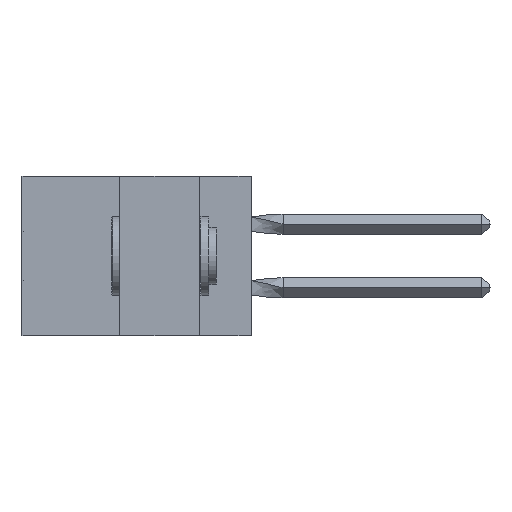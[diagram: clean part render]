
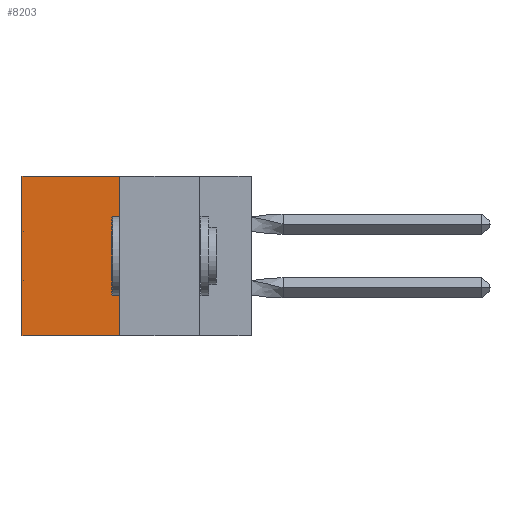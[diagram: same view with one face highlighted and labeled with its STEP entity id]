
A CAD part, left-side view. The second image highlights one B-rep face of the part: STEP entity #8203.
In plain terms, the highlighted planar face has unit normal (-1, 0, 0).
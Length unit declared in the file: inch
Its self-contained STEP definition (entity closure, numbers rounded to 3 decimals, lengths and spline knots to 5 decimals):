
#455 = VECTOR ( 'NONE', #11552, 39.37008 ) ;
#884 = CARTESIAN_POINT ( 'NONE',  ( 0.305, 0.72, -0.5 ) ) ;
#1140 = LINE ( 'NONE', #884, #28678 ) ;
#1660 = VERTEX_POINT ( 'NONE', #36398 ) ;
#2373 = EDGE_CURVE ( 'NONE', #28975, #3886, #28406, .T. ) ;
#2977 = DIRECTION ( 'NONE',  ( 1., 0., 0. ) ) ;
#3886 = VERTEX_POINT ( 'NONE', #41334 ) ;
#4423 = PLANE ( 'NONE',  #13043 ) ;
#5890 = DIRECTION ( 'NONE',  ( 0., 0., -1. ) ) ;
#8203 = ADVANCED_FACE ( 'NONE', ( #32040 ), #4423, .F. ) ;
#9246 = DIRECTION ( 'NONE',  ( 0., 1., 0. ) ) ;
#10403 = CARTESIAN_POINT ( 'NONE',  ( 0.305, 0.413, -0.5 ) ) ;
#11552 = DIRECTION ( 'NONE',  ( 0., 1., 0. ) ) ;
#13043 = AXIS2_PLACEMENT_3D ( 'NONE', #19679, #2977, #5890 ) ;
#13833 = VECTOR ( 'NONE', #9246, 39.37008 ) ;
#17580 = EDGE_CURVE ( 'NONE', #3886, #1660, #1140, .T. ) ;
#18030 = EDGE_LOOP ( 'NONE', ( #36988, #32866, #40586, #39161 ) ) ;
#18140 = LINE ( 'NONE', #10403, #455 ) ;
#18523 = VERTEX_POINT ( 'NONE', #29036 ) ;
#19679 = CARTESIAN_POINT ( 'NONE',  ( 0.305, 0.413, -0.5 ) ) ;
#22125 = CARTESIAN_POINT ( 'NONE',  ( 0.305, 0.413, -0.5 ) ) ;
#23223 = LINE ( 'NONE', #22125, #24782 ) ;
#24782 = VECTOR ( 'NONE', #32631, 39.37008 ) ;
#27350 = EDGE_CURVE ( 'NONE', #18523, #1660, #18140, .T. ) ;
#28406 = LINE ( 'NONE', #42436, #13833 ) ;
#28678 = VECTOR ( 'NONE', #30385, 39.37008 ) ;
#28975 = VERTEX_POINT ( 'NONE', #42535 ) ;
#29036 = CARTESIAN_POINT ( 'NONE',  ( 0.305, 0.413, -0.5 ) ) ;
#30385 = DIRECTION ( 'NONE',  ( 0., 0., -1. ) ) ;
#32040 = FACE_OUTER_BOUND ( 'NONE', #18030, .T. ) ;
#32631 = DIRECTION ( 'NONE',  ( 0., 0., -1. ) ) ;
#32866 = ORIENTED_EDGE ( 'NONE', *, *, #27350, .F. ) ;
#36398 = CARTESIAN_POINT ( 'NONE',  ( 0.305, 0.72, -0.5 ) ) ;
#36988 = ORIENTED_EDGE ( 'NONE', *, *, #17580, .T. ) ;
#39161 = ORIENTED_EDGE ( 'NONE', *, *, #2373, .T. ) ;
#40586 = ORIENTED_EDGE ( 'NONE', *, *, #42668, .F. ) ;
#41334 = CARTESIAN_POINT ( 'NONE',  ( 0.305, 0.72, 0. ) ) ;
#42436 = CARTESIAN_POINT ( 'NONE',  ( 0.305, 0.413, 0. ) ) ;
#42535 = CARTESIAN_POINT ( 'NONE',  ( 0.305, 0.413, 0. ) ) ;
#42668 = EDGE_CURVE ( 'NONE', #28975, #18523, #23223, .T. ) ;
